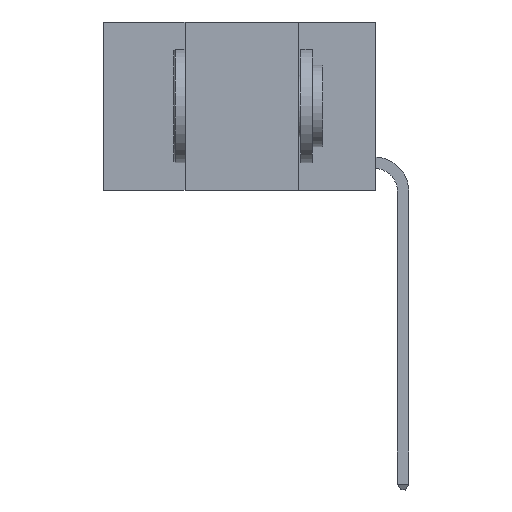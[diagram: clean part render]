
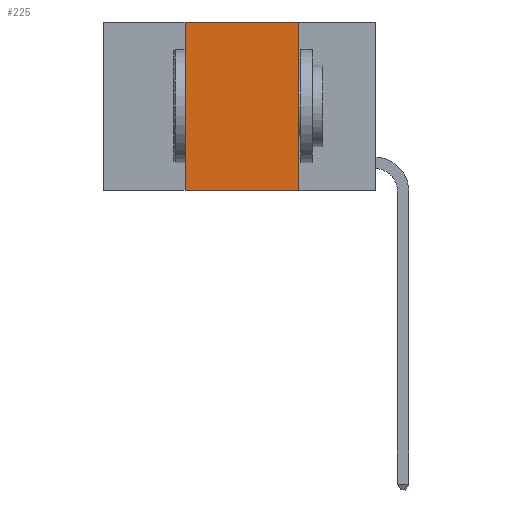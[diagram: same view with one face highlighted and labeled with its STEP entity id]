
A CAD part, left-side view. The second image highlights one B-rep face of the part: STEP entity #225.
In plain terms, the highlighted planar face has unit normal (-1, 0, 0).
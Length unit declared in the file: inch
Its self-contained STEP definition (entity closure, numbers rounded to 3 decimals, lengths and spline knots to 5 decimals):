
#141 = FACE_OUTER_BOUND ( 'NONE', #354, .T. ) ;
#225 = ADVANCED_FACE ( 'NONE', ( #141 ), #851, .F. ) ;
#354 = EDGE_LOOP ( 'NONE', ( #462, #7375, #691, #2500 ) ) ;
#413 = CARTESIAN_POINT ( 'NONE',  ( 0., 0.42, 0. ) ) ;
#462 = ORIENTED_EDGE ( 'NONE', *, *, #4132, .F. ) ;
#691 = ORIENTED_EDGE ( 'NONE', *, *, #7748, .F. ) ;
#793 = CARTESIAN_POINT ( 'NONE',  ( 0., 0.6, 0. ) ) ;
#849 = EDGE_CURVE ( 'NONE', #7540, #8543, #2995, .T. ) ;
#851 = PLANE ( 'NONE',  #7249 ) ;
#2331 = LINE ( 'NONE', #793, #7860 ) ;
#2464 = CARTESIAN_POINT ( 'NONE',  ( 0., 0.17, 0. ) ) ;
#2500 = ORIENTED_EDGE ( 'NONE', *, *, #849, .T. ) ;
#2557 = VECTOR ( 'NONE', #4664, 39.37008 ) ;
#2690 = CARTESIAN_POINT ( 'NONE',  ( 0., 0.17, 0. ) ) ;
#2995 = LINE ( 'NONE', #4400, #6548 ) ;
#3038 = DIRECTION ( 'NONE',  ( 0., -1., 0. ) ) ;
#3641 = LINE ( 'NONE', #2464, #9005 ) ;
#3948 = CARTESIAN_POINT ( 'NONE',  ( 0., 0.42, 0. ) ) ;
#4132 = EDGE_CURVE ( 'NONE', #8788, #8543, #3641, .T. ) ;
#4400 = CARTESIAN_POINT ( 'NONE',  ( 0., 0.6, -0.37 ) ) ;
#4619 = CARTESIAN_POINT ( 'NONE',  ( 0., 0.6, 0. ) ) ;
#4664 = DIRECTION ( 'NONE',  ( 0., 0., 1. ) ) ;
#5200 = CARTESIAN_POINT ( 'NONE',  ( 0., 0.42, -0.37 ) ) ;
#5294 = DIRECTION ( 'NONE',  ( 0., -1., 0. ) ) ;
#5389 = DIRECTION ( 'NONE',  ( 0., 0., -1. ) ) ;
#6123 = DIRECTION ( 'NONE',  ( 1., 0., 0. ) ) ;
#6263 = EDGE_CURVE ( 'NONE', #7396, #8788, #2331, .T. ) ;
#6548 = VECTOR ( 'NONE', #3038, 39.37008 ) ;
#7249 = AXIS2_PLACEMENT_3D ( 'NONE', #4619, #6123, #8568 ) ;
#7375 = ORIENTED_EDGE ( 'NONE', *, *, #6263, .F. ) ;
#7396 = VERTEX_POINT ( 'NONE', #413 ) ;
#7540 = VERTEX_POINT ( 'NONE', #5200 ) ;
#7748 = EDGE_CURVE ( 'NONE', #7540, #7396, #8275, .T. ) ;
#7860 = VECTOR ( 'NONE', #5294, 39.37008 ) ;
#8275 = LINE ( 'NONE', #3948, #2557 ) ;
#8543 = VERTEX_POINT ( 'NONE', #8785 ) ;
#8568 = DIRECTION ( 'NONE',  ( 0., 0., -1. ) ) ;
#8785 = CARTESIAN_POINT ( 'NONE',  ( 0., 0.17, -0.37 ) ) ;
#8788 = VERTEX_POINT ( 'NONE', #2690 ) ;
#9005 = VECTOR ( 'NONE', #5389, 39.37008 ) ;
